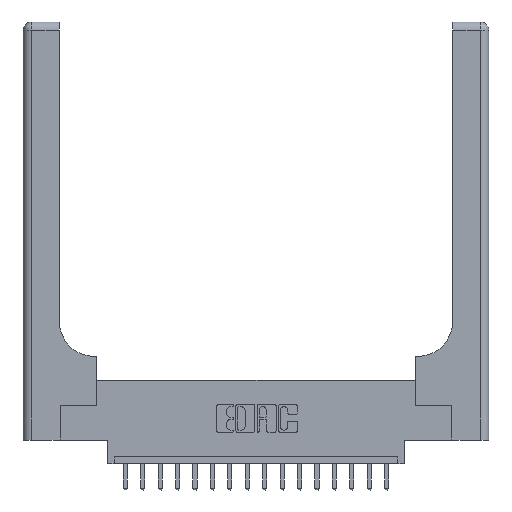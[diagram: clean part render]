
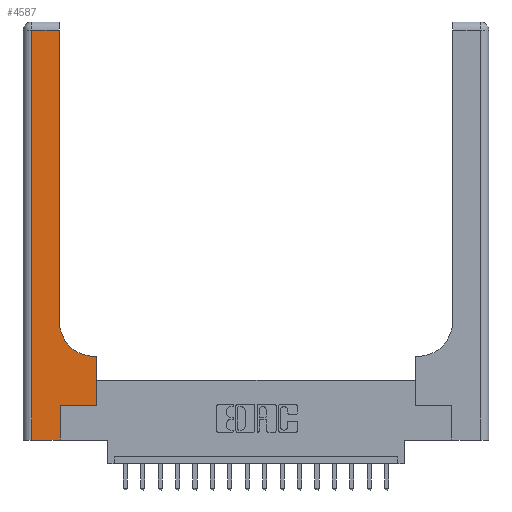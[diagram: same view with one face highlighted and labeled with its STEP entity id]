
A CAD part, top view. The second image highlights one B-rep face of the part: STEP entity #4587.
In plain terms, the highlighted planar face has unit normal (0, 0, 1).
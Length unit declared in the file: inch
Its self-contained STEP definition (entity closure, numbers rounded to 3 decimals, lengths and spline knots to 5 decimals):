
#192 = EDGE_CURVE ( 'NONE', #9385, #10744, #14885, .T. ) ;
#211 = VERTEX_POINT ( 'NONE', #3859 ) ;
#221 = ORIENTED_EDGE ( 'NONE', *, *, #8135, .T. ) ;
#701 = DIRECTION ( 'NONE',  ( 1., 0., 0. ) ) ;
#1231 = LINE ( 'NONE', #2603, #1725 ) ;
#1459 = DIRECTION ( 'NONE',  ( -1., 0., 0. ) ) ;
#1582 = VERTEX_POINT ( 'NONE', #14506 ) ;
#1725 = VECTOR ( 'NONE', #5416, 39.37008 ) ;
#1803 = LINE ( 'NONE', #7710, #3539 ) ;
#1999 = VERTEX_POINT ( 'NONE', #14488 ) ;
#2114 = VECTOR ( 'NONE', #9948, 39.37008 ) ;
#2603 = CARTESIAN_POINT ( 'NONE',  ( 0., 0., 0.37 ) ) ;
#2764 = ORIENTED_EDGE ( 'NONE', *, *, #14466, .T. ) ;
#2988 = CARTESIAN_POINT ( 'NONE',  ( 0.51, 0.85, 0.37 ) ) ;
#3491 = EDGE_LOOP ( 'NONE', ( #11512, #9403, #11864, #13686, #6299, #2764, #4008, #221, #13240 ) ) ;
#3539 = VECTOR ( 'NONE', #5331, 39.37008 ) ;
#3827 = DIRECTION ( 'NONE',  ( -1., 0., 0. ) ) ;
#3859 = CARTESIAN_POINT ( 'NONE',  ( 0.51, 0.6, 0.37 ) ) ;
#4008 = ORIENTED_EDGE ( 'NONE', *, *, #15309, .T. ) ;
#4587 = ADVANCED_FACE ( 'NONE', ( #9204 ), #8830, .F. ) ;
#4740 = EDGE_CURVE ( 'NONE', #1582, #9385, #1231, .T. ) ;
#5177 = CARTESIAN_POINT ( 'NONE',  ( 0.26, 2.94, 0.37 ) ) ;
#5331 = DIRECTION ( 'NONE',  ( 0., -1., 0. ) ) ;
#5416 = DIRECTION ( 'NONE',  ( 1., 0., 0. ) ) ;
#5684 = CARTESIAN_POINT ( 'NONE',  ( 0.26, 3., 0.37 ) ) ;
#5991 = DIRECTION ( 'NONE',  ( 0., 1., 0. ) ) ;
#6275 = CARTESIAN_POINT ( 'NONE',  ( 0.528, 0.25, 0.37 ) ) ;
#6299 = ORIENTED_EDGE ( 'NONE', *, *, #192, .T. ) ;
#6583 = VECTOR ( 'NONE', #701, 39.37008 ) ;
#6596 = DIRECTION ( 'NONE',  ( 0., 1., 0. ) ) ;
#6704 = VECTOR ( 'NONE', #13433, 39.37008 ) ;
#6882 = AXIS2_PLACEMENT_3D ( 'NONE', #2988, #11934, #8899 ) ;
#7554 = EDGE_CURVE ( 'NONE', #12454, #11140, #11428, .T. ) ;
#7710 = CARTESIAN_POINT ( 'NONE',  ( 0.06, 3., 0.37 ) ) ;
#8003 = CARTESIAN_POINT ( 'NONE',  ( 0.265, 0., 0.37 ) ) ;
#8056 = VECTOR ( 'NONE', #5991, 39.37008 ) ;
#8135 = EDGE_CURVE ( 'NONE', #1999, #211, #11024, .T. ) ;
#8231 = LINE ( 'NONE', #9288, #13449 ) ;
#8830 = PLANE ( 'NONE',  #9446 ) ;
#8899 = DIRECTION ( 'NONE',  ( 1., 0., 0. ) ) ;
#9204 = FACE_OUTER_BOUND ( 'NONE', #3491, .T. ) ;
#9288 = CARTESIAN_POINT ( 'NONE',  ( 0.528, 0.25, 0.37 ) ) ;
#9308 = VERTEX_POINT ( 'NONE', #6275 ) ;
#9340 = CARTESIAN_POINT ( 'NONE',  ( 0.06, 2.94, 0.37 ) ) ;
#9385 = VERTEX_POINT ( 'NONE', #8003 ) ;
#9403 = ORIENTED_EDGE ( 'NONE', *, *, #11788, .T. ) ;
#9446 = AXIS2_PLACEMENT_3D ( 'NONE', #14814, #13435, #1459 ) ;
#9948 = DIRECTION ( 'NONE',  ( 0., 1., 0. ) ) ;
#10032 = CARTESIAN_POINT ( 'NONE',  ( 0.265, 0.25, 0.37 ) ) ;
#10744 = VERTEX_POINT ( 'NONE', #10032 ) ;
#10913 = LINE ( 'NONE', #18837, #6583 ) ;
#11024 = LINE ( 'NONE', #17005, #15209 ) ;
#11140 = VERTEX_POINT ( 'NONE', #5177 ) ;
#11229 = CIRCLE ( 'NONE', #6882, 0.25 ) ;
#11242 = CARTESIAN_POINT ( 'NONE',  ( 0.26, 0.85, 0.37 ) ) ;
#11428 = LINE ( 'NONE', #5684, #2114 ) ;
#11512 = ORIENTED_EDGE ( 'NONE', *, *, #7554, .T. ) ;
#11788 = EDGE_CURVE ( 'NONE', #11140, #15651, #14813, .T. ) ;
#11864 = ORIENTED_EDGE ( 'NONE', *, *, #12119, .T. ) ;
#11934 = DIRECTION ( 'NONE',  ( 0., 0., -1. ) ) ;
#12119 = EDGE_CURVE ( 'NONE', #15651, #1582, #1803, .T. ) ;
#12454 = VERTEX_POINT ( 'NONE', #11242 ) ;
#13240 = ORIENTED_EDGE ( 'NONE', *, *, #13836, .T. ) ;
#13335 = CARTESIAN_POINT ( 'NONE',  ( 0., 2.94, 0.37 ) ) ;
#13433 = DIRECTION ( 'NONE',  ( -1., 0., 0. ) ) ;
#13435 = DIRECTION ( 'NONE',  ( 0., 0., -1. ) ) ;
#13449 = VECTOR ( 'NONE', #6596, 39.37008 ) ;
#13686 = ORIENTED_EDGE ( 'NONE', *, *, #4740, .T. ) ;
#13836 = EDGE_CURVE ( 'NONE', #211, #12454, #11229, .T. ) ;
#14466 = EDGE_CURVE ( 'NONE', #10744, #9308, #10913, .T. ) ;
#14488 = CARTESIAN_POINT ( 'NONE',  ( 0.528, 0.6, 0.37 ) ) ;
#14506 = CARTESIAN_POINT ( 'NONE',  ( 0.06, 0., 0.37 ) ) ;
#14813 = LINE ( 'NONE', #13335, #6704 ) ;
#14814 = CARTESIAN_POINT ( 'NONE',  ( 0., 3., 0.37 ) ) ;
#14885 = LINE ( 'NONE', #17800, #8056 ) ;
#15209 = VECTOR ( 'NONE', #3827, 39.37008 ) ;
#15309 = EDGE_CURVE ( 'NONE', #9308, #1999, #8231, .T. ) ;
#15651 = VERTEX_POINT ( 'NONE', #9340 ) ;
#17005 = CARTESIAN_POINT ( 'NONE',  ( 0.26, 0.6, 0.37 ) ) ;
#17800 = CARTESIAN_POINT ( 'NONE',  ( 0.265, 0., 0.37 ) ) ;
#18837 = CARTESIAN_POINT ( 'NONE',  ( 0.265, 0.25, 0.37 ) ) ;
